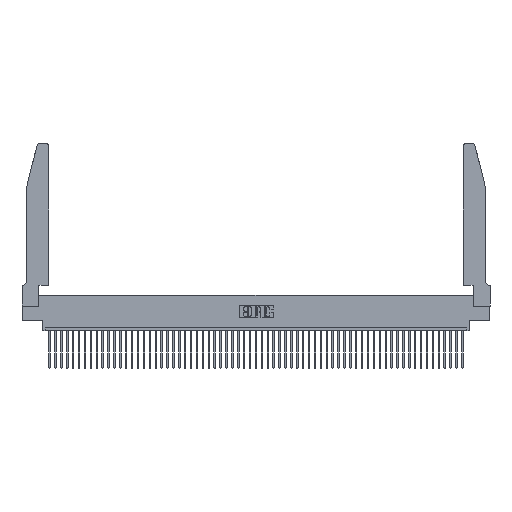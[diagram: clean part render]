
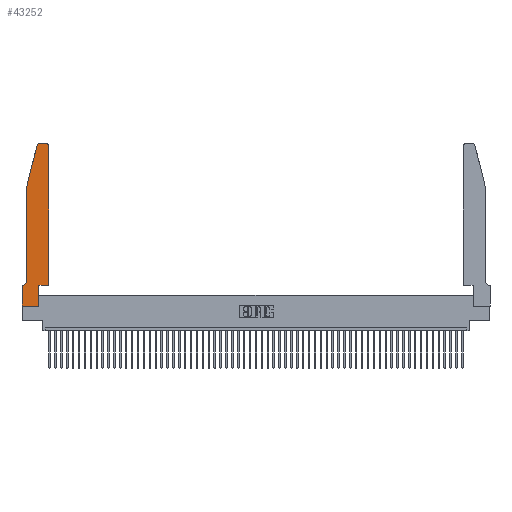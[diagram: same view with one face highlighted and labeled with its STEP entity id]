
A CAD part, top view. The second image highlights one B-rep face of the part: STEP entity #43252.
In plain terms, the highlighted planar face has unit normal (0, 0, 1).
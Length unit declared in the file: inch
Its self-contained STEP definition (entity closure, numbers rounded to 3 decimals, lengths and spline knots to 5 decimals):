
#564 = ORIENTED_EDGE ( 'NONE', *, *, #37373, .T. ) ;
#722 = EDGE_CURVE ( 'NONE', #11429, #45131, #34560, .T. ) ;
#1117 = VERTEX_POINT ( 'NONE', #7215 ) ;
#1198 = EDGE_CURVE ( 'NONE', #21342, #12119, #12903, .T. ) ;
#1690 = CARTESIAN_POINT ( 'NONE',  ( 0.2605, 2.75, 0.37 ) ) ;
#1809 = AXIS2_PLACEMENT_3D ( 'NONE', #39280, #22202, #26778 ) ;
#2511 = CARTESIAN_POINT ( 'NONE',  ( 0.0755, 0.42, 0.37 ) ) ;
#2913 = EDGE_CURVE ( 'NONE', #50272, #11429, #20039, .T. ) ;
#4453 = AXIS2_PLACEMENT_3D ( 'NONE', #35242, #22188, #9361 ) ;
#4623 = LINE ( 'NONE', #1690, #10518 ) ;
#4979 = CARTESIAN_POINT ( 'NONE',  ( 0.4505, 0.35, 0.37 ) ) ;
#5346 = AXIS2_PLACEMENT_3D ( 'NONE', #13215, #38701, #22158 ) ;
#6915 = AXIS2_PLACEMENT_3D ( 'NONE', #41559, #16430, #7785 ) ;
#7096 = LINE ( 'NONE', #38163, #20952 ) ;
#7215 = CARTESIAN_POINT ( 'NONE',  ( 0.2865, 0.35, 0.37 ) ) ;
#7785 = DIRECTION ( 'NONE',  ( 1., 0., 0. ) ) ;
#8133 = VERTEX_POINT ( 'NONE', #34782 ) ;
#8157 = VERTEX_POINT ( 'NONE', #48344 ) ;
#8363 = LINE ( 'NONE', #42842, #17455 ) ;
#8575 = ORIENTED_EDGE ( 'NONE', *, *, #35348, .T. ) ;
#8600 = ORIENTED_EDGE ( 'NONE', *, *, #16863, .T. ) ;
#9103 = CARTESIAN_POINT ( 'NONE',  ( 0.2865, 0.35, 0.37 ) ) ;
#9361 = DIRECTION ( 'NONE',  ( 1., 0., 0. ) ) ;
#10276 = VERTEX_POINT ( 'NONE', #24408 ) ;
#10518 = VECTOR ( 'NONE', #52441, 39.37008 ) ;
#11429 = VERTEX_POINT ( 'NONE', #2511 ) ;
#11798 = FACE_OUTER_BOUND ( 'NONE', #21953, .T. ) ;
#12119 = VERTEX_POINT ( 'NONE', #47974 ) ;
#12227 = ORIENTED_EDGE ( 'NONE', *, *, #48949, .T. ) ;
#12556 = DIRECTION ( 'NONE',  ( -0.239, -0.971, 0. ) ) ;
#12756 = LINE ( 'NONE', #4979, #52737 ) ;
#12903 = CIRCLE ( 'NONE', #6915, 0.03 ) ;
#13215 = CARTESIAN_POINT ( 'NONE',  ( 0., 0.35, 0.37 ) ) ;
#13398 = VECTOR ( 'NONE', #38473, 39.37008 ) ;
#13470 = DIRECTION ( 'NONE',  ( 1., 0., 0. ) ) ;
#13779 = CARTESIAN_POINT ( 'NONE',  ( 0.25487, 2.72718, 0.37 ) ) ;
#14340 = VERTEX_POINT ( 'NONE', #37091 ) ;
#14727 = DIRECTION ( 'NONE',  ( 1., 0., 0. ) ) ;
#15868 = ORIENTED_EDGE ( 'NONE', *, *, #28858, .T. ) ;
#16253 = CARTESIAN_POINT ( 'NONE',  ( 0.0755, 2., 0.37 ) ) ;
#16430 = DIRECTION ( 'NONE',  ( 0., 0., 1. ) ) ;
#16863 = EDGE_CURVE ( 'NONE', #12119, #8133, #4623, .T. ) ;
#16960 = CARTESIAN_POINT ( 'NONE',  ( 0.2865, 0., 0.37 ) ) ;
#17455 = VECTOR ( 'NONE', #14727, 39.37008 ) ;
#18461 = LINE ( 'NONE', #32965, #24481 ) ;
#20039 = LINE ( 'NONE', #16253, #47444 ) ;
#20952 = VECTOR ( 'NONE', #29864, 39.37008 ) ;
#20981 = VECTOR ( 'NONE', #31594, 39.37008 ) ;
#21342 = VERTEX_POINT ( 'NONE', #29900 ) ;
#21584 = LINE ( 'NONE', #26619, #20981 ) ;
#21953 = EDGE_LOOP ( 'NONE', ( #8600, #30968, #48299, #29180, #32128, #12227, #8575, #24261, #564, #49680, #15868, #53278 ) ) ;
#22158 = DIRECTION ( 'NONE',  ( 1., 0., 0. ) ) ;
#22188 = DIRECTION ( 'NONE',  ( 0., 0., 1. ) ) ;
#22202 = DIRECTION ( 'NONE',  ( 0., 0., -1. ) ) ;
#22861 = VECTOR ( 'NONE', #52479, 39.37008 ) ;
#24261 = ORIENTED_EDGE ( 'NONE', *, *, #38508, .T. ) ;
#24408 = CARTESIAN_POINT ( 'NONE',  ( 0., 0.35, 0.37 ) ) ;
#24481 = VECTOR ( 'NONE', #12556, 39.37008 ) ;
#25804 = CARTESIAN_POINT ( 'NONE',  ( 0.4505, 0.35, 0.37 ) ) ;
#26619 = CARTESIAN_POINT ( 'NONE',  ( 0.0755, 0.35, 0.37 ) ) ;
#26778 = DIRECTION ( 'NONE',  ( -1., 0., 0. ) ) ;
#28858 = EDGE_CURVE ( 'NONE', #8157, #21342, #34099, .T. ) ;
#29180 = ORIENTED_EDGE ( 'NONE', *, *, #2913, .T. ) ;
#29456 = CARTESIAN_POINT ( 'NONE',  ( 0.0755, 2., 0.37 ) ) ;
#29864 = DIRECTION ( 'NONE',  ( 0., -1., 0. ) ) ;
#29900 = CARTESIAN_POINT ( 'NONE',  ( 0.4505, 2.72, 0.37 ) ) ;
#30968 = ORIENTED_EDGE ( 'NONE', *, *, #37941, .T. ) ;
#31594 = DIRECTION ( 'NONE',  ( -1., 0., 0. ) ) ;
#32128 = ORIENTED_EDGE ( 'NONE', *, *, #722, .T. ) ;
#32965 = CARTESIAN_POINT ( 'NONE',  ( 0.0755, 2., 0.37 ) ) ;
#34099 = LINE ( 'NONE', #25804, #22861 ) ;
#34560 = CIRCLE ( 'NONE', #1809, 0.07 ) ;
#34664 = PLANE ( 'NONE',  #5346 ) ;
#34782 = CARTESIAN_POINT ( 'NONE',  ( 0.284, 2.75, 0.37 ) ) ;
#35242 = CARTESIAN_POINT ( 'NONE',  ( 0.284, 2.72, 0.37 ) ) ;
#35348 = EDGE_CURVE ( 'NONE', #10276, #14340, #7096, .T. ) ;
#37091 = CARTESIAN_POINT ( 'NONE',  ( 0., 0., 0.37 ) ) ;
#37373 = EDGE_CURVE ( 'NONE', #47363, #1117, #42948, .T. ) ;
#37941 = EDGE_CURVE ( 'NONE', #8133, #40468, #52701, .T. ) ;
#38163 = CARTESIAN_POINT ( 'NONE',  ( 0., 0., 0.37 ) ) ;
#38473 = DIRECTION ( 'NONE',  ( 0., 1., 0. ) ) ;
#38508 = EDGE_CURVE ( 'NONE', #14340, #47363, #8363, .T. ) ;
#38701 = DIRECTION ( 'NONE',  ( 0., 0., 1. ) ) ;
#39280 = CARTESIAN_POINT ( 'NONE',  ( 0.0055, 0.42, 0.37 ) ) ;
#40468 = VERTEX_POINT ( 'NONE', #13779 ) ;
#41559 = CARTESIAN_POINT ( 'NONE',  ( 0.4205, 2.72, 0.37 ) ) ;
#42842 = CARTESIAN_POINT ( 'NONE',  ( 0., 0., 0.37 ) ) ;
#42948 = LINE ( 'NONE', #9103, #13398 ) ;
#43252 = ADVANCED_FACE ( 'NONE', ( #11798 ), #34664, .T. ) ;
#45131 = VERTEX_POINT ( 'NONE', #52980 ) ;
#45628 = DIRECTION ( 'NONE',  ( 0., -1., 0. ) ) ;
#45646 = EDGE_CURVE ( 'NONE', #1117, #8157, #12756, .T. ) ;
#46491 = EDGE_CURVE ( 'NONE', #40468, #50272, #18461, .T. ) ;
#47363 = VERTEX_POINT ( 'NONE', #16960 ) ;
#47444 = VECTOR ( 'NONE', #45628, 39.37008 ) ;
#47974 = CARTESIAN_POINT ( 'NONE',  ( 0.4205, 2.75, 0.37 ) ) ;
#48299 = ORIENTED_EDGE ( 'NONE', *, *, #46491, .T. ) ;
#48344 = CARTESIAN_POINT ( 'NONE',  ( 0.4505, 0.35, 0.37 ) ) ;
#48949 = EDGE_CURVE ( 'NONE', #45131, #10276, #21584, .T. ) ;
#49680 = ORIENTED_EDGE ( 'NONE', *, *, #45646, .T. ) ;
#50272 = VERTEX_POINT ( 'NONE', #29456 ) ;
#52441 = DIRECTION ( 'NONE',  ( -1., 0., 0. ) ) ;
#52479 = DIRECTION ( 'NONE',  ( 0., 1., 0. ) ) ;
#52701 = CIRCLE ( 'NONE', #4453, 0.03 ) ;
#52737 = VECTOR ( 'NONE', #13470, 39.37008 ) ;
#52980 = CARTESIAN_POINT ( 'NONE',  ( 0.0055, 0.35, 0.37 ) ) ;
#53278 = ORIENTED_EDGE ( 'NONE', *, *, #1198, .T. ) ;
